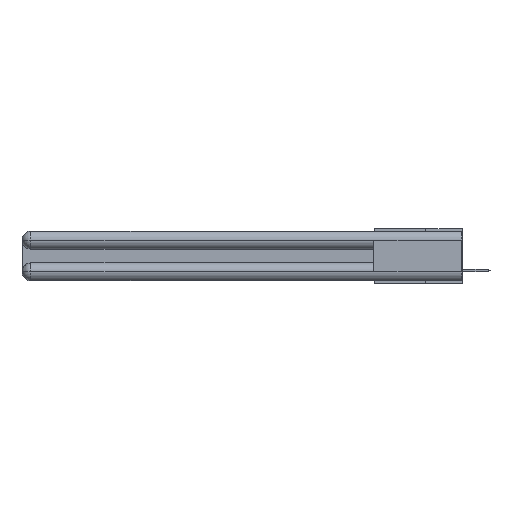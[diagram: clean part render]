
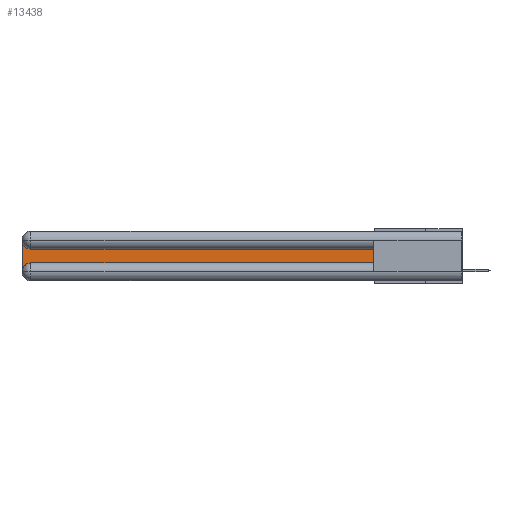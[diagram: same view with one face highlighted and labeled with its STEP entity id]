
A CAD part, left-side view. The second image highlights one B-rep face of the part: STEP entity #13438.
In plain terms, the highlighted planar face has unit normal (-1, 0, 0).
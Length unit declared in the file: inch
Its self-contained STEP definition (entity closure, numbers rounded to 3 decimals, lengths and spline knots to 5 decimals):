
#541 = CARTESIAN_POINT ( 'NONE',  ( 0.075, 0.6, -0.1225 ) ) ;
#2716 = CARTESIAN_POINT ( 'NONE',  ( 0.075, 3., -0.0625 ) ) ;
#2823 = CARTESIAN_POINT ( 'NONE',  ( 0.075, 2.94, -0.1225 ) ) ;
#3953 = ORIENTED_EDGE ( 'NONE', *, *, #25973, .T. ) ;
#4087 = DIRECTION ( 'NONE',  ( 0., -1., 0. ) ) ;
#4220 = AXIS2_PLACEMENT_3D ( 'NONE', #28415, #26282, #19232 ) ;
#5258 = DIRECTION ( 'NONE',  ( 0., 1., 0. ) ) ;
#6101 = CARTESIAN_POINT ( 'NONE',  ( 0.075, 2.94, -0.0625 ) ) ;
#6353 = CARTESIAN_POINT ( 'NONE',  ( 0.075, 0.6, -0.2175 ) ) ;
#6542 = EDGE_LOOP ( 'NONE', ( #28529, #25878, #3953, #23149, #20172, #7352 ) ) ;
#7314 = VECTOR ( 'NONE', #11405, 39.37008 ) ;
#7352 = ORIENTED_EDGE ( 'NONE', *, *, #16676, .T. ) ;
#7610 = CARTESIAN_POINT ( 'NONE',  ( 0.075, 2.94, -0.2175 ) ) ;
#7858 = EDGE_CURVE ( 'NONE', #22490, #13104, #13090, .T. ) ;
#8053 = VERTEX_POINT ( 'NONE', #23237 ) ;
#8061 = VERTEX_POINT ( 'NONE', #2716 ) ;
#8174 = EDGE_CURVE ( 'NONE', #27345, #17408, #25690, .T. ) ;
#8371 = DIRECTION ( 'NONE',  ( 0., 0., -1. ) ) ;
#8747 = LINE ( 'NONE', #26501, #24564 ) ;
#9153 = CARTESIAN_POINT ( 'NONE',  ( 0.075, 0.6, -0.2175 ) ) ;
#9267 = CARTESIAN_POINT ( 'NONE',  ( 0.075, 0.6, -0.1225 ) ) ;
#11124 = AXIS2_PLACEMENT_3D ( 'NONE', #6101, #21830, #8371 ) ;
#11405 = DIRECTION ( 'NONE',  ( 0., 0., 1. ) ) ;
#11638 = VECTOR ( 'NONE', #5258, 39.37008 ) ;
#11771 = CIRCLE ( 'NONE', #11124, 0.06 ) ;
#13090 = LINE ( 'NONE', #6353, #27112 ) ;
#13104 = VERTEX_POINT ( 'NONE', #17770 ) ;
#13438 = ADVANCED_FACE ( 'NONE', ( #26654 ), #15107, .F. ) ;
#15107 = PLANE ( 'NONE',  #4220 ) ;
#15340 = DIRECTION ( 'NONE',  ( 0., 0., -1. ) ) ;
#16448 = LINE ( 'NONE', #9153, #7314 ) ;
#16676 = EDGE_CURVE ( 'NONE', #13104, #27345, #16448, .T. ) ;
#17408 = VERTEX_POINT ( 'NONE', #2823 ) ;
#17770 = CARTESIAN_POINT ( 'NONE',  ( 0.075, 0.6, -0.2175 ) ) ;
#18489 = EDGE_CURVE ( 'NONE', #17408, #8061, #11771, .T. ) ;
#19232 = DIRECTION ( 'NONE',  ( 0., 0., -1. ) ) ;
#19916 = CARTESIAN_POINT ( 'NONE',  ( 0.075, 2.94, -0.2775 ) ) ;
#20172 = ORIENTED_EDGE ( 'NONE', *, *, #7858, .T. ) ;
#21830 = DIRECTION ( 'NONE',  ( 1., 0., 0. ) ) ;
#22168 = DIRECTION ( 'NONE',  ( 0., 0., -1. ) ) ;
#22490 = VERTEX_POINT ( 'NONE', #7610 ) ;
#23149 = ORIENTED_EDGE ( 'NONE', *, *, #26553, .T. ) ;
#23237 = CARTESIAN_POINT ( 'NONE',  ( 0.075, 3., -0.2775 ) ) ;
#23467 = CIRCLE ( 'NONE', #24405, 0.06 ) ;
#24405 = AXIS2_PLACEMENT_3D ( 'NONE', #19916, #26861, #22168 ) ;
#24564 = VECTOR ( 'NONE', #15340, 39.37008 ) ;
#25690 = LINE ( 'NONE', #541, #11638 ) ;
#25878 = ORIENTED_EDGE ( 'NONE', *, *, #18489, .T. ) ;
#25973 = EDGE_CURVE ( 'NONE', #8061, #8053, #8747, .T. ) ;
#26282 = DIRECTION ( 'NONE',  ( 1., 0., 0. ) ) ;
#26501 = CARTESIAN_POINT ( 'NONE',  ( 0.075, 3., -0.2175 ) ) ;
#26553 = EDGE_CURVE ( 'NONE', #8053, #22490, #23467, .T. ) ;
#26654 = FACE_OUTER_BOUND ( 'NONE', #6542, .T. ) ;
#26861 = DIRECTION ( 'NONE',  ( 1., 0., 0. ) ) ;
#27112 = VECTOR ( 'NONE', #4087, 39.37008 ) ;
#27345 = VERTEX_POINT ( 'NONE', #9267 ) ;
#28415 = CARTESIAN_POINT ( 'NONE',  ( 0.075, 3., -0.1225 ) ) ;
#28529 = ORIENTED_EDGE ( 'NONE', *, *, #8174, .T. ) ;
